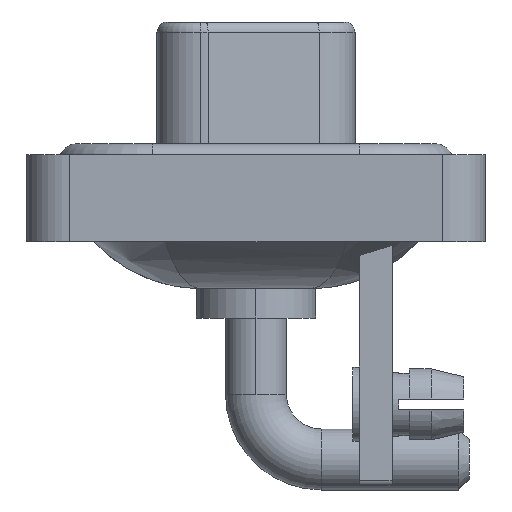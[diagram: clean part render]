
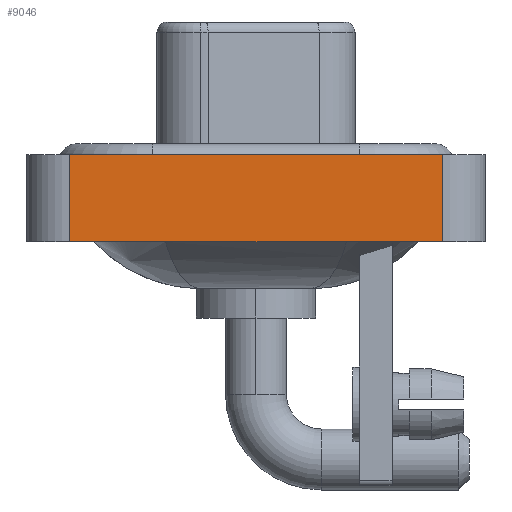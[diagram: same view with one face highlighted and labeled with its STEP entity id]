
A CAD part, left-side view. The second image highlights one B-rep face of the part: STEP entity #9046.
In plain terms, the highlighted planar face has unit normal (-1, 0, 0).
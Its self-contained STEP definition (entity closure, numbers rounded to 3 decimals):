
#125 = ORIENTED_EDGE ( 'NONE', *, *, #15685, .F. ) ;
#534 = ORIENTED_EDGE ( 'NONE', *, *, #18216, .F. ) ;
#576 = VERTEX_POINT ( 'NONE', #5928 ) ;
#1728 = CARTESIAN_POINT ( 'NONE',  ( -7.3, -8.55, -3.6 ) ) ;
#2972 = EDGE_CURVE ( 'NONE', #576, #3575, #4410, .T. ) ;
#3156 = FACE_OUTER_BOUND ( 'NONE', #8345, .T. ) ;
#3575 = VERTEX_POINT ( 'NONE', #6625 ) ;
#3740 = ORIENTED_EDGE ( 'NONE', *, *, #2972, .T. ) ;
#4238 = VECTOR ( 'NONE', #16075, 1000. ) ;
#4364 = CARTESIAN_POINT ( 'NONE',  ( -7.3, 8.55, -3.6 ) ) ;
#4410 = LINE ( 'NONE', #10251, #4238 ) ;
#5928 = CARTESIAN_POINT ( 'NONE',  ( -7.3, -8.55, -3.6 ) ) ;
#5987 = VECTOR ( 'NONE', #10611, 1000. ) ;
#6065 = PLANE ( 'NONE',  #6619 ) ;
#6619 = AXIS2_PLACEMENT_3D ( 'NONE', #1728, #14672, #16195 ) ;
#6625 = CARTESIAN_POINT ( 'NONE',  ( -7.3, -8.55, 0.4 ) ) ;
#7241 = LINE ( 'NONE', #4364, #14809 ) ;
#8345 = EDGE_LOOP ( 'NONE', ( #3740, #534, #125, #13470 ) ) ;
#8782 = VECTOR ( 'NONE', #15978, 1000. ) ;
#9046 = ADVANCED_FACE ( 'NONE', ( #3156 ), #6065, .T. ) ;
#9711 = CARTESIAN_POINT ( 'NONE',  ( -7.3, 8.55, 0.4 ) ) ;
#10251 = CARTESIAN_POINT ( 'NONE',  ( -7.3, -8.55, -3.6 ) ) ;
#10430 = LINE ( 'NONE', #14921, #5987 ) ;
#10611 = DIRECTION ( 'NONE',  ( 0., -1., 0. ) ) ;
#11314 = VERTEX_POINT ( 'NONE', #18798 ) ;
#11337 = EDGE_CURVE ( 'NONE', #11314, #576, #10430, .T. ) ;
#12776 = VERTEX_POINT ( 'NONE', #9711 ) ;
#13470 = ORIENTED_EDGE ( 'NONE', *, *, #11337, .T. ) ;
#14672 = DIRECTION ( 'NONE',  ( -1., 0., 0. ) ) ;
#14704 = DIRECTION ( 'NONE',  ( 0., 0., 1. ) ) ;
#14809 = VECTOR ( 'NONE', #14704, 1000. ) ;
#14921 = CARTESIAN_POINT ( 'NONE',  ( -7.3, -8.55, -3.6 ) ) ;
#15685 = EDGE_CURVE ( 'NONE', #11314, #12776, #7241, .T. ) ;
#15978 = DIRECTION ( 'NONE',  ( 0., -1., 0. ) ) ;
#16075 = DIRECTION ( 'NONE',  ( 0., 0., 1. ) ) ;
#16195 = DIRECTION ( 'NONE',  ( 0., 0., 1. ) ) ;
#17502 = CARTESIAN_POINT ( 'NONE',  ( -7.3, -8.55, 0.4 ) ) ;
#18216 = EDGE_CURVE ( 'NONE', #12776, #3575, #18834, .T. ) ;
#18798 = CARTESIAN_POINT ( 'NONE',  ( -7.3, 8.55, -3.6 ) ) ;
#18834 = LINE ( 'NONE', #17502, #8782 ) ;
